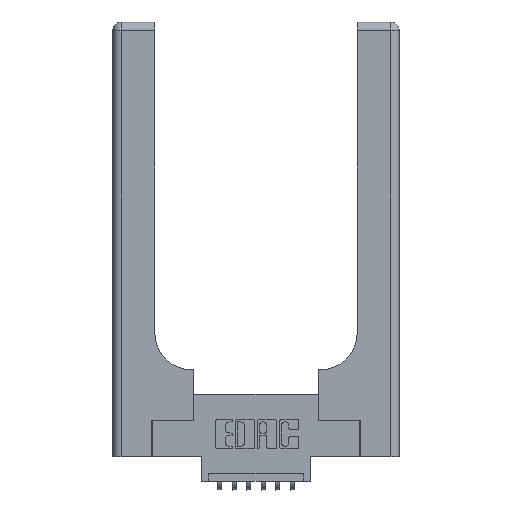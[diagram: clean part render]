
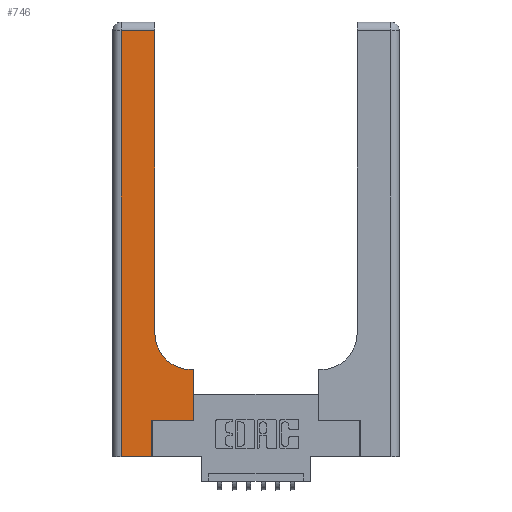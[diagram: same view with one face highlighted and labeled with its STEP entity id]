
A CAD part, top view. The second image highlights one B-rep face of the part: STEP entity #746.
In plain terms, the highlighted planar face has unit normal (0, 0, 1).
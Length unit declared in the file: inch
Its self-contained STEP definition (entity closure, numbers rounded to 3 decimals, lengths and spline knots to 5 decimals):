
#43 = LINE ( 'NONE', #10896, #5727 ) ;
#611 = CARTESIAN_POINT ( 'NONE',  ( 0.2915, 0.6, 0.37 ) ) ;
#746 = ADVANCED_FACE ( 'NONE', ( #5462 ), #3656, .F. ) ;
#1445 = DIRECTION ( 'NONE',  ( 0., -1., 0. ) ) ;
#1865 = LINE ( 'NONE', #2767, #6102 ) ;
#1964 = DIRECTION ( 'NONE',  ( 0., 1., 0. ) ) ;
#1967 = ORIENTED_EDGE ( 'NONE', *, *, #4110, .T. ) ;
#2014 = VERTEX_POINT ( 'NONE', #11407 ) ;
#2564 = CARTESIAN_POINT ( 'NONE',  ( 0.269, 0., 0.37 ) ) ;
#2767 = CARTESIAN_POINT ( 'NONE',  ( 0., 2.94, 0.37 ) ) ;
#2926 = LINE ( 'NONE', #2564, #14680 ) ;
#2971 = CARTESIAN_POINT ( 'NONE',  ( 0.2915, 0.85, 0.37 ) ) ;
#3073 = LINE ( 'NONE', #7355, #4837 ) ;
#3181 = EDGE_LOOP ( 'NONE', ( #10063, #7009, #13887, #1967, #9927, #11984, #14505, #4665, #6323 ) ) ;
#3445 = LINE ( 'NONE', #9384, #8840 ) ;
#3656 = PLANE ( 'NONE',  #9162 ) ;
#3817 = CARTESIAN_POINT ( 'NONE',  ( 0.269, 0., 0.37 ) ) ;
#4110 = EDGE_CURVE ( 'NONE', #13718, #13269, #43, .T. ) ;
#4144 = EDGE_CURVE ( 'NONE', #14084, #12835, #3073, .T. ) ;
#4171 = CIRCLE ( 'NONE', #12959, 0.25 ) ;
#4613 = VERTEX_POINT ( 'NONE', #13544 ) ;
#4665 = ORIENTED_EDGE ( 'NONE', *, *, #9777, .T. ) ;
#4679 = DIRECTION ( 'NONE',  ( 0., 1., 0. ) ) ;
#4837 = VECTOR ( 'NONE', #4925, 39.37008 ) ;
#4925 = DIRECTION ( 'NONE',  ( 0., 1., 0. ) ) ;
#4990 = EDGE_CURVE ( 'NONE', #9090, #14084, #4171, .T. ) ;
#5462 = FACE_OUTER_BOUND ( 'NONE', #3181, .T. ) ;
#5727 = VECTOR ( 'NONE', #12947, 39.37008 ) ;
#5841 = EDGE_CURVE ( 'NONE', #2014, #13718, #3445, .T. ) ;
#5888 = CARTESIAN_POINT ( 'NONE',  ( 0., 3., 0.37 ) ) ;
#5909 = CARTESIAN_POINT ( 'NONE',  ( 0.269, 0.25, 0.37 ) ) ;
#5942 = DIRECTION ( 'NONE',  ( -1., 0., 0. ) ) ;
#6022 = LINE ( 'NONE', #611, #6911 ) ;
#6095 = CARTESIAN_POINT ( 'NONE',  ( 0.5415, 0.6, 0.37 ) ) ;
#6102 = VECTOR ( 'NONE', #10757, 39.37008 ) ;
#6148 = DIRECTION ( 'NONE',  ( -1., 0., 0. ) ) ;
#6323 = ORIENTED_EDGE ( 'NONE', *, *, #4990, .T. ) ;
#6387 = CARTESIAN_POINT ( 'NONE',  ( 0.5585, 0.25, 0.37 ) ) ;
#6572 = CARTESIAN_POINT ( 'NONE',  ( 0.5415, 0.85, 0.37 ) ) ;
#6650 = EDGE_CURVE ( 'NONE', #13269, #4613, #2926, .T. ) ;
#6792 = VECTOR ( 'NONE', #11582, 39.37008 ) ;
#6911 = VECTOR ( 'NONE', #6148, 39.37008 ) ;
#7009 = ORIENTED_EDGE ( 'NONE', *, *, #12652, .T. ) ;
#7133 = VERTEX_POINT ( 'NONE', #13723 ) ;
#7355 = CARTESIAN_POINT ( 'NONE',  ( 0.2915, 3., 0.37 ) ) ;
#7754 = DIRECTION ( 'NONE',  ( 0., 0., -1. ) ) ;
#8840 = VECTOR ( 'NONE', #1445, 39.37008 ) ;
#9090 = VERTEX_POINT ( 'NONE', #6095 ) ;
#9162 = AXIS2_PLACEMENT_3D ( 'NONE', #5888, #12806, #5942 ) ;
#9384 = CARTESIAN_POINT ( 'NONE',  ( 0.06, 3., 0.37 ) ) ;
#9777 = EDGE_CURVE ( 'NONE', #12847, #9090, #6022, .T. ) ;
#9927 = ORIENTED_EDGE ( 'NONE', *, *, #6650, .T. ) ;
#10053 = CARTESIAN_POINT ( 'NONE',  ( 0.5585, 0.6, 0.37 ) ) ;
#10063 = ORIENTED_EDGE ( 'NONE', *, *, #4144, .T. ) ;
#10757 = DIRECTION ( 'NONE',  ( -1., 0., 0. ) ) ;
#10896 = CARTESIAN_POINT ( 'NONE',  ( 0., 0., 0.37 ) ) ;
#10927 = EDGE_CURVE ( 'NONE', #7133, #12847, #11377, .T. ) ;
#11202 = DIRECTION ( 'NONE',  ( 1., 0., 0. ) ) ;
#11293 = LINE ( 'NONE', #5909, #6792 ) ;
#11377 = LINE ( 'NONE', #6387, #11923 ) ;
#11407 = CARTESIAN_POINT ( 'NONE',  ( 0.06, 2.94, 0.37 ) ) ;
#11582 = DIRECTION ( 'NONE',  ( 1., 0., 0. ) ) ;
#11923 = VECTOR ( 'NONE', #1964, 39.37008 ) ;
#11984 = ORIENTED_EDGE ( 'NONE', *, *, #13137, .T. ) ;
#12498 = CARTESIAN_POINT ( 'NONE',  ( 0.06, 0., 0.37 ) ) ;
#12652 = EDGE_CURVE ( 'NONE', #12835, #2014, #1865, .T. ) ;
#12806 = DIRECTION ( 'NONE',  ( 0., 0., -1. ) ) ;
#12835 = VERTEX_POINT ( 'NONE', #14376 ) ;
#12847 = VERTEX_POINT ( 'NONE', #10053 ) ;
#12947 = DIRECTION ( 'NONE',  ( 1., 0., 0. ) ) ;
#12959 = AXIS2_PLACEMENT_3D ( 'NONE', #6572, #7754, #11202 ) ;
#13137 = EDGE_CURVE ( 'NONE', #4613, #7133, #11293, .T. ) ;
#13269 = VERTEX_POINT ( 'NONE', #3817 ) ;
#13544 = CARTESIAN_POINT ( 'NONE',  ( 0.269, 0.25, 0.37 ) ) ;
#13718 = VERTEX_POINT ( 'NONE', #12498 ) ;
#13723 = CARTESIAN_POINT ( 'NONE',  ( 0.5585, 0.25, 0.37 ) ) ;
#13887 = ORIENTED_EDGE ( 'NONE', *, *, #5841, .T. ) ;
#14084 = VERTEX_POINT ( 'NONE', #2971 ) ;
#14376 = CARTESIAN_POINT ( 'NONE',  ( 0.2915, 2.94, 0.37 ) ) ;
#14505 = ORIENTED_EDGE ( 'NONE', *, *, #10927, .T. ) ;
#14680 = VECTOR ( 'NONE', #4679, 39.37008 ) ;
